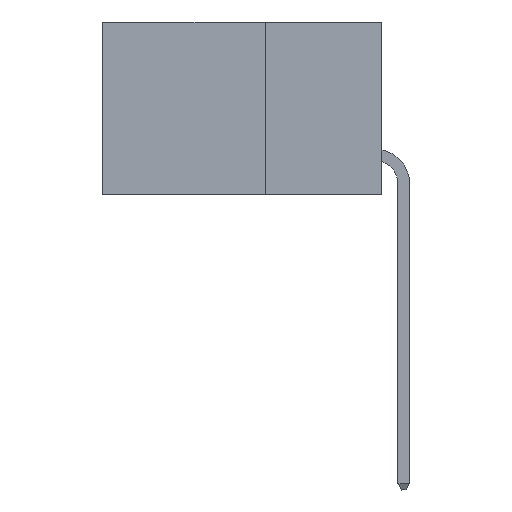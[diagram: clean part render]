
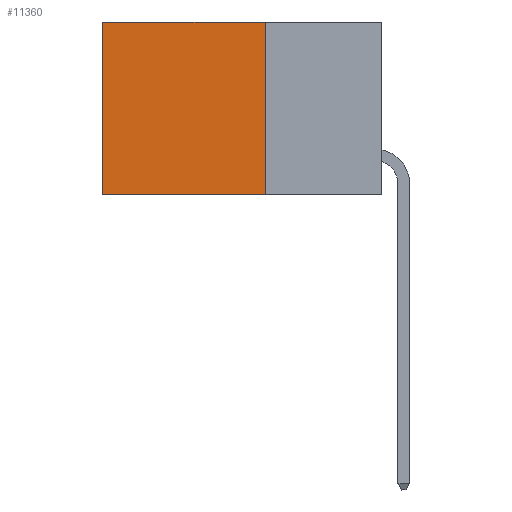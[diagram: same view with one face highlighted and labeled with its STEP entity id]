
A CAD part, left-side view. The second image highlights one B-rep face of the part: STEP entity #11360.
In plain terms, the highlighted planar face has unit normal (-1, 0, 0).
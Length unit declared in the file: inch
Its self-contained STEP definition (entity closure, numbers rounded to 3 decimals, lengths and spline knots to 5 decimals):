
#552 = VERTEX_POINT ( 'NONE', #22383 ) ;
#2204 = CARTESIAN_POINT ( 'NONE',  ( 0.2875, 0.25, 0. ) ) ;
#2294 = ORIENTED_EDGE ( 'NONE', *, *, #21554, .F. ) ;
#2359 = EDGE_LOOP ( 'NONE', ( #22113, #2294, #13470, #14311 ) ) ;
#2943 = FACE_OUTER_BOUND ( 'NONE', #2359, .T. ) ;
#2990 = VECTOR ( 'NONE', #8552, 39.37008 ) ;
#3087 = LINE ( 'NONE', #18362, #21982 ) ;
#3264 = PLANE ( 'NONE',  #19395 ) ;
#4231 = VECTOR ( 'NONE', #20529, 39.37008 ) ;
#5344 = LINE ( 'NONE', #11806, #4231 ) ;
#5608 = EDGE_CURVE ( 'NONE', #12896, #21615, #12460, .T. ) ;
#5876 = DIRECTION ( 'NONE',  ( 0., 1., 0. ) ) ;
#6155 = DIRECTION ( 'NONE',  ( 0., 0., -1. ) ) ;
#6412 = DIRECTION ( 'NONE',  ( 0., 0., -1. ) ) ;
#7908 = CARTESIAN_POINT ( 'NONE',  ( 0.2875, 0.25, 0. ) ) ;
#8552 = DIRECTION ( 'NONE',  ( 0., 1., 0. ) ) ;
#8665 = EDGE_CURVE ( 'NONE', #12896, #23015, #3087, .T. ) ;
#9358 = DIRECTION ( 'NONE',  ( 1., 0., 0. ) ) ;
#10326 = CARTESIAN_POINT ( 'NONE',  ( 0.2875, 0.25, -0.37 ) ) ;
#11360 = ADVANCED_FACE ( 'NONE', ( #2943 ), #3264, .F. ) ;
#11806 = CARTESIAN_POINT ( 'NONE',  ( 0.2875, 0.6, 0. ) ) ;
#12460 = LINE ( 'NONE', #7908, #12744 ) ;
#12744 = VECTOR ( 'NONE', #6412, 39.37008 ) ;
#12896 = VERTEX_POINT ( 'NONE', #17664 ) ;
#13470 = ORIENTED_EDGE ( 'NONE', *, *, #5608, .F. ) ;
#14139 = CARTESIAN_POINT ( 'NONE',  ( 0.2875, 0.6, 0. ) ) ;
#14311 = ORIENTED_EDGE ( 'NONE', *, *, #8665, .T. ) ;
#17664 = CARTESIAN_POINT ( 'NONE',  ( 0.2875, 0.25, 0. ) ) ;
#18118 = EDGE_CURVE ( 'NONE', #23015, #552, #5344, .T. ) ;
#18362 = CARTESIAN_POINT ( 'NONE',  ( 0.2875, 0.25, 0. ) ) ;
#18539 = LINE ( 'NONE', #19235, #2990 ) ;
#19235 = CARTESIAN_POINT ( 'NONE',  ( 0.2875, 0.25, -0.37 ) ) ;
#19395 = AXIS2_PLACEMENT_3D ( 'NONE', #2204, #9358, #6155 ) ;
#20529 = DIRECTION ( 'NONE',  ( 0., 0., -1. ) ) ;
#21554 = EDGE_CURVE ( 'NONE', #21615, #552, #18539, .T. ) ;
#21615 = VERTEX_POINT ( 'NONE', #10326 ) ;
#21982 = VECTOR ( 'NONE', #5876, 39.37008 ) ;
#22113 = ORIENTED_EDGE ( 'NONE', *, *, #18118, .T. ) ;
#22383 = CARTESIAN_POINT ( 'NONE',  ( 0.2875, 0.6, -0.37 ) ) ;
#23015 = VERTEX_POINT ( 'NONE', #14139 ) ;
